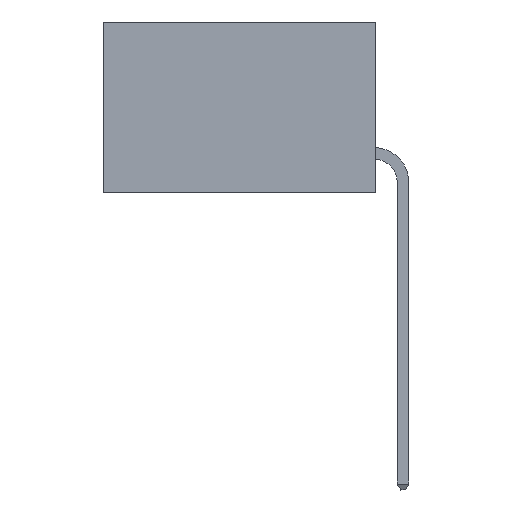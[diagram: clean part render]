
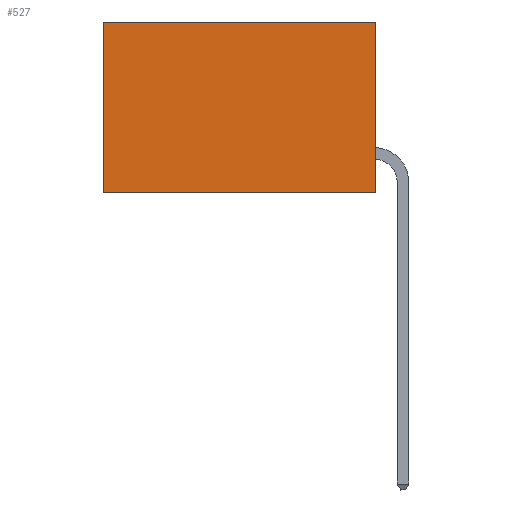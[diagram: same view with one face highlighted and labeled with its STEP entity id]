
A CAD part, left-side view. The second image highlights one B-rep face of the part: STEP entity #527.
In plain terms, the highlighted planar face has unit normal (-1, 0, 0).
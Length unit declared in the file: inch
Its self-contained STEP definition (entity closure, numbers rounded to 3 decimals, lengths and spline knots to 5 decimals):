
#527 = ADVANCED_FACE ( 'NONE', ( #5219 ), #23445, .F. ) ;
#1420 = VERTEX_POINT ( 'NONE', #10708 ) ;
#1563 = DIRECTION ( 'NONE',  ( 0., 1., 0. ) ) ;
#1696 = ORIENTED_EDGE ( 'NONE', *, *, #7678, .T. ) ;
#1808 = CARTESIAN_POINT ( 'NONE',  ( 0.277, 0., 0. ) ) ;
#2398 = EDGE_CURVE ( 'NONE', #20867, #1420, #16246, .T. ) ;
#2626 = DIRECTION ( 'NONE',  ( 0., 1., 0. ) ) ;
#3396 = LINE ( 'NONE', #10421, #13132 ) ;
#3476 = VECTOR ( 'NONE', #1563, 39.37008 ) ;
#4236 = EDGE_CURVE ( 'NONE', #24823, #1420, #3396, .T. ) ;
#4323 = CARTESIAN_POINT ( 'NONE',  ( 0.277, 0., -0.37 ) ) ;
#4400 = VERTEX_POINT ( 'NONE', #7317 ) ;
#5219 = FACE_OUTER_BOUND ( 'NONE', #10619, .T. ) ;
#7317 = CARTESIAN_POINT ( 'NONE',  ( 0.277, 0., 0. ) ) ;
#7525 = CARTESIAN_POINT ( 'NONE',  ( 0.277, 0.59, 0. ) ) ;
#7529 = LINE ( 'NONE', #17248, #17149 ) ;
#7678 = EDGE_CURVE ( 'NONE', #4400, #24823, #8706, .T. ) ;
#8706 = LINE ( 'NONE', #1808, #3476 ) ;
#9621 = CARTESIAN_POINT ( 'NONE',  ( 0.277, 0., -0.37 ) ) ;
#9850 = ORIENTED_EDGE ( 'NONE', *, *, #4236, .T. ) ;
#10298 = AXIS2_PLACEMENT_3D ( 'NONE', #9621, #21424, #13189 ) ;
#10421 = CARTESIAN_POINT ( 'NONE',  ( 0.277, 0.59, -0.37 ) ) ;
#10619 = EDGE_LOOP ( 'NONE', ( #9850, #23265, #12738, #1696 ) ) ;
#10708 = CARTESIAN_POINT ( 'NONE',  ( 0.277, 0.59, -0.37 ) ) ;
#10790 = DIRECTION ( 'NONE',  ( 0., 0., -1. ) ) ;
#12738 = ORIENTED_EDGE ( 'NONE', *, *, #14249, .F. ) ;
#13132 = VECTOR ( 'NONE', #10790, 39.37008 ) ;
#13189 = DIRECTION ( 'NONE',  ( 0., 0., -1. ) ) ;
#13759 = CARTESIAN_POINT ( 'NONE',  ( 0.277, 0., -0.37 ) ) ;
#14249 = EDGE_CURVE ( 'NONE', #4400, #20867, #7529, .T. ) ;
#16246 = LINE ( 'NONE', #4323, #20086 ) ;
#17149 = VECTOR ( 'NONE', #19141, 39.37008 ) ;
#17248 = CARTESIAN_POINT ( 'NONE',  ( 0.277, 0., -0.37 ) ) ;
#19141 = DIRECTION ( 'NONE',  ( 0., 0., -1. ) ) ;
#20086 = VECTOR ( 'NONE', #2626, 39.37008 ) ;
#20867 = VERTEX_POINT ( 'NONE', #13759 ) ;
#21424 = DIRECTION ( 'NONE',  ( 1., 0., 0. ) ) ;
#23265 = ORIENTED_EDGE ( 'NONE', *, *, #2398, .F. ) ;
#23445 = PLANE ( 'NONE',  #10298 ) ;
#24823 = VERTEX_POINT ( 'NONE', #7525 ) ;
